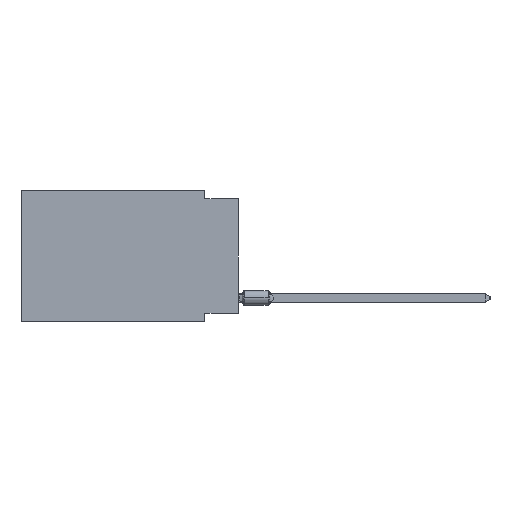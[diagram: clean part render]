
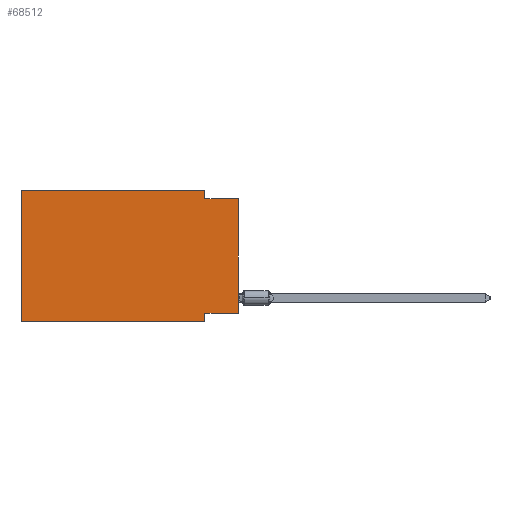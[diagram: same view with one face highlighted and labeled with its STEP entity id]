
A CAD part, left-side view. The second image highlights one B-rep face of the part: STEP entity #68512.
In plain terms, the highlighted planar face has unit normal (-1, 0, 0).
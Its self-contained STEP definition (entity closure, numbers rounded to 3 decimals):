
#48 = VECTOR ( 'NONE', #62035, 1000. ) ;
#1325 = VERTEX_POINT ( 'NONE', #62345 ) ;
#2314 = LINE ( 'NONE', #67373, #47692 ) ;
#2340 = ORIENTED_EDGE ( 'NONE', *, *, #13846, .F. ) ;
#2396 = LINE ( 'NONE', #29073, #68435 ) ;
#4993 = DIRECTION ( 'NONE',  ( 0., 0., -1. ) ) ;
#9042 = LINE ( 'NONE', #52083, #48 ) ;
#9088 = ORIENTED_EDGE ( 'NONE', *, *, #58214, .T. ) ;
#11930 = DIRECTION ( 'NONE',  ( 0., 0., -1. ) ) ;
#12977 = EDGE_LOOP ( 'NONE', ( #9088, #43366, #60163, #2340, #38200, #28902, #49505, #38912 ) ) ;
#13846 = EDGE_CURVE ( 'NONE', #28326, #1325, #9042, .T. ) ;
#14723 = CARTESIAN_POINT ( 'NONE',  ( 0., 2.54, -9.271 ) ) ;
#14853 = LINE ( 'NONE', #58239, #41206 ) ;
#15049 = VERTEX_POINT ( 'NONE', #14723 ) ;
#15165 = CARTESIAN_POINT ( 'NONE',  ( 0., 0., -9.271 ) ) ;
#16021 = CARTESIAN_POINT ( 'NONE',  ( 0., 0., -9.271 ) ) ;
#16396 = DIRECTION ( 'NONE',  ( 0., 0., 1. ) ) ;
#18956 = LINE ( 'NONE', #61630, #49842 ) ;
#19658 = VECTOR ( 'NONE', #68621, 1000. ) ;
#19926 = VERTEX_POINT ( 'NONE', #15165 ) ;
#20048 = CARTESIAN_POINT ( 'NONE',  ( 0., 2.54, -0.635 ) ) ;
#22758 = EDGE_CURVE ( 'NONE', #65853, #28326, #65107, .T. ) ;
#23247 = DIRECTION ( 'NONE',  ( 0., -1., 0. ) ) ;
#23381 = DIRECTION ( 'NONE',  ( 0., -1., 0. ) ) ;
#28326 = VERTEX_POINT ( 'NONE', #37909 ) ;
#28902 = ORIENTED_EDGE ( 'NONE', *, *, #51719, .T. ) ;
#29073 = CARTESIAN_POINT ( 'NONE',  ( 0., 0., -0.635 ) ) ;
#29824 = EDGE_CURVE ( 'NONE', #1325, #54118, #2314, .T. ) ;
#34864 = EDGE_CURVE ( 'NONE', #54118, #62248, #2396, .T. ) ;
#35577 = CARTESIAN_POINT ( 'NONE',  ( 0., 0., 0. ) ) ;
#37024 = EDGE_CURVE ( 'NONE', #19926, #15049, #48030, .T. ) ;
#37909 = CARTESIAN_POINT ( 'NONE',  ( 0., 16.383, 0. ) ) ;
#38200 = ORIENTED_EDGE ( 'NONE', *, *, #22758, .F. ) ;
#38393 = CARTESIAN_POINT ( 'NONE',  ( 0., 0., -0.635 ) ) ;
#38912 = ORIENTED_EDGE ( 'NONE', *, *, #37024, .F. ) ;
#39182 = CARTESIAN_POINT ( 'NONE',  ( 0., 16.383, -9.906 ) ) ;
#41206 = VECTOR ( 'NONE', #47921, 1000. ) ;
#41390 = VERTEX_POINT ( 'NONE', #44716 ) ;
#41649 = PLANE ( 'NONE',  #49980 ) ;
#41997 = CARTESIAN_POINT ( 'NONE',  ( 0., 16.383, 0. ) ) ;
#43366 = ORIENTED_EDGE ( 'NONE', *, *, #34864, .F. ) ;
#44716 = CARTESIAN_POINT ( 'NONE',  ( 0., 2.54, -9.906 ) ) ;
#47692 = VECTOR ( 'NONE', #11930, 1000. ) ;
#47921 = DIRECTION ( 'NONE',  ( 0., 0., -1. ) ) ;
#48030 = LINE ( 'NONE', #16021, #64249 ) ;
#49505 = ORIENTED_EDGE ( 'NONE', *, *, #55848, .F. ) ;
#49842 = VECTOR ( 'NONE', #23247, 1000. ) ;
#49980 = AXIS2_PLACEMENT_3D ( 'NONE', #41997, #63322, #4993 ) ;
#51719 = EDGE_CURVE ( 'NONE', #65853, #41390, #18956, .T. ) ;
#52083 = CARTESIAN_POINT ( 'NONE',  ( 0., 16.383, 0. ) ) ;
#52787 = VECTOR ( 'NONE', #16396, 1000. ) ;
#54060 = FACE_OUTER_BOUND ( 'NONE', #12977, .T. ) ;
#54118 = VERTEX_POINT ( 'NONE', #20048 ) ;
#55848 = EDGE_CURVE ( 'NONE', #15049, #41390, #14853, .T. ) ;
#57043 = DIRECTION ( 'NONE',  ( 0., 1., 0. ) ) ;
#58214 = EDGE_CURVE ( 'NONE', #19926, #62248, #69326, .T. ) ;
#58239 = CARTESIAN_POINT ( 'NONE',  ( 0., 2.54, -9.906 ) ) ;
#59779 = CARTESIAN_POINT ( 'NONE',  ( 0., 16.383, 0. ) ) ;
#60163 = ORIENTED_EDGE ( 'NONE', *, *, #29824, .F. ) ;
#61630 = CARTESIAN_POINT ( 'NONE',  ( 0., 16.383, -9.906 ) ) ;
#62035 = DIRECTION ( 'NONE',  ( 0., -1., 0. ) ) ;
#62248 = VERTEX_POINT ( 'NONE', #38393 ) ;
#62345 = CARTESIAN_POINT ( 'NONE',  ( 0., 2.54, 0. ) ) ;
#63322 = DIRECTION ( 'NONE',  ( 1., 0., 0. ) ) ;
#64249 = VECTOR ( 'NONE', #57043, 1000. ) ;
#65107 = LINE ( 'NONE', #59779, #52787 ) ;
#65853 = VERTEX_POINT ( 'NONE', #39182 ) ;
#67373 = CARTESIAN_POINT ( 'NONE',  ( 0., 2.54, 0. ) ) ;
#68435 = VECTOR ( 'NONE', #23381, 1000. ) ;
#68512 = ADVANCED_FACE ( 'NONE', ( #54060 ), #41649, .F. ) ;
#68621 = DIRECTION ( 'NONE',  ( 0., 0., 1. ) ) ;
#69326 = LINE ( 'NONE', #35577, #19658 ) ;
